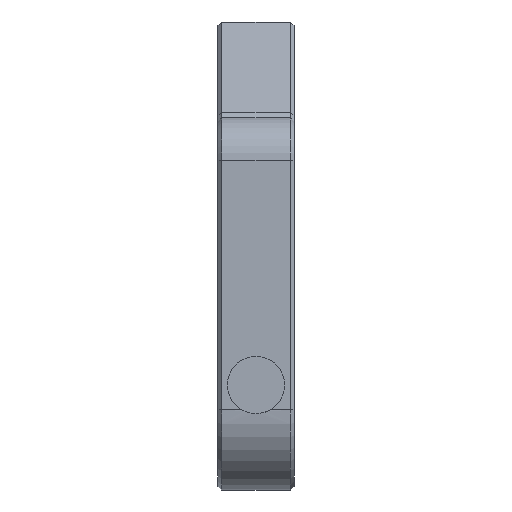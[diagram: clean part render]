
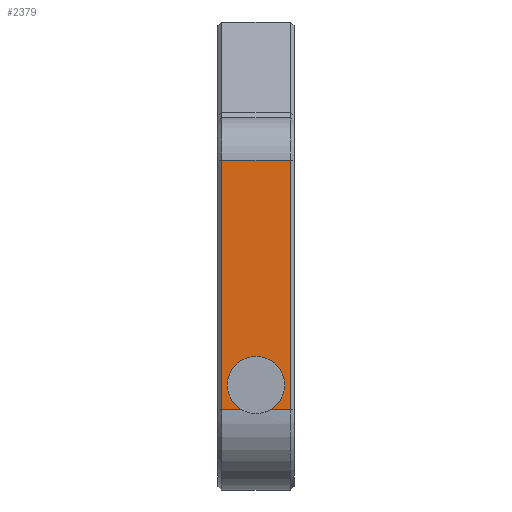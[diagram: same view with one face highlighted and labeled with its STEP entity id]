
A CAD part, left-side view. The second image highlights one B-rep face of the part: STEP entity #2379.
In plain terms, the highlighted planar face has unit normal (-1, 0, 0).
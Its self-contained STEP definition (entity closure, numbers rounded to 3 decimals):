
#224 = PLANE('',#225);
#225 = AXIS2_PLACEMENT_3D('',#226,#227,#228);
#226 = CARTESIAN_POINT('',(11.2,-3.8,-28.5));
#227 = DIRECTION('',(0.707,0.707,0.));
#228 = DIRECTION('',(0.,0.,-1.));
#1197 = VERTEX_POINT('',#1198);
#1198 = CARTESIAN_POINT('',(11.,-3.6,-28.5));
#1232 = CYLINDRICAL_SURFACE('',#1233,4.5);
#1233 = AXIS2_PLACEMENT_3D('',#1234,#1235,#1236);
#1234 = CARTESIAN_POINT('',(15.5,-4.,-28.5));
#1235 = DIRECTION('',(0.,1.,0.));
#1236 = DIRECTION('',(-1.,0.,0.));
#1303 = VERTEX_POINT('',#1304);
#1304 = CARTESIAN_POINT('',(11.,-3.6,-54.6));
#1323 = EDGE_CURVE('',#1197,#1303,#1324,.T.);
#1324 = SURFACE_CURVE('',#1325,(#1329,#1336),.PCURVE_S1.);
#1325 = LINE('',#1326,#1327);
#1326 = CARTESIAN_POINT('',(11.,-3.6,-28.5));
#1327 = VECTOR('',#1328,1.);
#1328 = DIRECTION('',(-0.,-0.,-1.));
#1329 = PCURVE('',#224,#1330);
#1330 = DEFINITIONAL_REPRESENTATION('',(#1331),#1335);
#1331 = LINE('',#1332,#1333);
#1332 = CARTESIAN_POINT('',(0.,0.283));
#1333 = VECTOR('',#1334,1.);
#1334 = DIRECTION('',(1.,0.));
#1335 = ( GEOMETRIC_REPRESENTATION_CONTEXT(2) 
PARAMETRIC_REPRESENTATION_CONTEXT() REPRESENTATION_CONTEXT('2D SPACE',''
  ) );
#1336 = PCURVE('',#1337,#1342);
#1337 = PLANE('',#1338);
#1338 = AXIS2_PLACEMENT_3D('',#1339,#1340,#1341);
#1339 = CARTESIAN_POINT('',(11.,-4.,-63.));
#1340 = DIRECTION('',(1.,0.,0.));
#1341 = DIRECTION('',(0.,0.,1.));
#1342 = DEFINITIONAL_REPRESENTATION('',(#1343),#1347);
#1343 = LINE('',#1344,#1345);
#1344 = CARTESIAN_POINT('',(34.5,-0.4));
#1345 = VECTOR('',#1346,1.);
#1346 = DIRECTION('',(-1.,0.));
#1347 = ( GEOMETRIC_REPRESENTATION_CONTEXT(2) 
PARAMETRIC_REPRESENTATION_CONTEXT() REPRESENTATION_CONTEXT('2D SPACE',''
  ) );
#1443 = CYLINDRICAL_SURFACE('',#1444,8.4);
#1444 = AXIS2_PLACEMENT_3D('',#1445,#1446,#1447);
#1445 = CARTESIAN_POINT('',(19.4,-4.,-54.6));
#1446 = DIRECTION('',(0.,1.,0.));
#1447 = DIRECTION('',(0.,0.,-1.));
#2275 = VERTEX_POINT('',#2276);
#2276 = CARTESIAN_POINT('',(11.,3.6,-28.5));
#2303 = EDGE_CURVE('',#1197,#2275,#2304,.T.);
#2304 = SURFACE_CURVE('',#2305,(#2309,#2316),.PCURVE_S1.);
#2305 = LINE('',#2306,#2307);
#2306 = CARTESIAN_POINT('',(11.,-4.,-28.5));
#2307 = VECTOR('',#2308,1.);
#2308 = DIRECTION('',(0.,1.,0.));
#2309 = PCURVE('',#1232,#2310);
#2310 = DEFINITIONAL_REPRESENTATION('',(#2311),#2315);
#2311 = LINE('',#2312,#2313);
#2312 = CARTESIAN_POINT('',(0.,0.));
#2313 = VECTOR('',#2314,1.);
#2314 = DIRECTION('',(0.,1.));
#2315 = ( GEOMETRIC_REPRESENTATION_CONTEXT(2) 
PARAMETRIC_REPRESENTATION_CONTEXT() REPRESENTATION_CONTEXT('2D SPACE',''
  ) );
#2316 = PCURVE('',#1337,#2317);
#2317 = DEFINITIONAL_REPRESENTATION('',(#2318),#2322);
#2318 = LINE('',#2319,#2320);
#2319 = CARTESIAN_POINT('',(34.5,0.));
#2320 = VECTOR('',#2321,1.);
#2321 = DIRECTION('',(0.,-1.));
#2322 = ( GEOMETRIC_REPRESENTATION_CONTEXT(2) 
PARAMETRIC_REPRESENTATION_CONTEXT() REPRESENTATION_CONTEXT('2D SPACE',''
  ) );
#2379 = ADVANCED_FACE('',(#2380),#1337,.F.);
#2380 = FACE_BOUND('',#2381,.F.);
#2381 = EDGE_LOOP('',(#2382,#2383,#2384,#2407,#2440,#2463));
#2382 = ORIENTED_EDGE('',*,*,#2303,.F.);
#2383 = ORIENTED_EDGE('',*,*,#1323,.T.);
#2384 = ORIENTED_EDGE('',*,*,#2385,.T.);
#2385 = EDGE_CURVE('',#1303,#2386,#2388,.T.);
#2386 = VERTEX_POINT('',#2387);
#2387 = CARTESIAN_POINT('',(11.,-1.497,-54.6));
#2388 = SURFACE_CURVE('',#2389,(#2393,#2400),.PCURVE_S1.);
#2389 = LINE('',#2390,#2391);
#2390 = CARTESIAN_POINT('',(11.,-4.,-54.6));
#2391 = VECTOR('',#2392,1.);
#2392 = DIRECTION('',(0.,1.,0.));
#2393 = PCURVE('',#1337,#2394);
#2394 = DEFINITIONAL_REPRESENTATION('',(#2395),#2399);
#2395 = LINE('',#2396,#2397);
#2396 = CARTESIAN_POINT('',(8.4,0.));
#2397 = VECTOR('',#2398,1.);
#2398 = DIRECTION('',(0.,-1.));
#2399 = ( GEOMETRIC_REPRESENTATION_CONTEXT(2) 
PARAMETRIC_REPRESENTATION_CONTEXT() REPRESENTATION_CONTEXT('2D SPACE',''
  ) );
#2400 = PCURVE('',#1443,#2401);
#2401 = DEFINITIONAL_REPRESENTATION('',(#2402),#2406);
#2402 = LINE('',#2403,#2404);
#2403 = CARTESIAN_POINT('',(1.571,0.));
#2404 = VECTOR('',#2405,1.);
#2405 = DIRECTION('',(0.,1.));
#2406 = ( GEOMETRIC_REPRESENTATION_CONTEXT(2) 
PARAMETRIC_REPRESENTATION_CONTEXT() REPRESENTATION_CONTEXT('2D SPACE',''
  ) );
#2407 = ORIENTED_EDGE('',*,*,#2408,.T.);
#2408 = EDGE_CURVE('',#2386,#2409,#2411,.T.);
#2409 = VERTEX_POINT('',#2410);
#2410 = CARTESIAN_POINT('',(11.,1.497,-54.6));
#2411 = SURFACE_CURVE('',#2412,(#2417,#2428),.PCURVE_S1.);
#2412 = CIRCLE('',#2413,3.);
#2413 = AXIS2_PLACEMENT_3D('',#2414,#2415,#2416);
#2414 = CARTESIAN_POINT('',(11.,0.,-52.));
#2415 = DIRECTION('',(-1.,-0.,0.));
#2416 = DIRECTION('',(0.,0.,-1.));
#2417 = PCURVE('',#1337,#2418);
#2418 = DEFINITIONAL_REPRESENTATION('',(#2419),#2427);
#2419 = ( BOUNDED_CURVE() B_SPLINE_CURVE(2,(#2420,#2421,#2422,#2423,
#2424,#2425,#2426),.UNSPECIFIED.,.T.,.F.) B_SPLINE_CURVE_WITH_KNOTS((1,2
    ,2,2,2,1),(-2.094,0.,2.094,4.189,
6.283,8.378),.UNSPECIFIED.) CURVE() 
GEOMETRIC_REPRESENTATION_ITEM() RATIONAL_B_SPLINE_CURVE((1.,0.5,1.,0.5,
1.,0.5,1.)) REPRESENTATION_ITEM('') );
#2420 = CARTESIAN_POINT('',(8.,-4.));
#2421 = CARTESIAN_POINT('',(8.,1.196));
#2422 = CARTESIAN_POINT('',(12.5,-1.402));
#2423 = CARTESIAN_POINT('',(17.,-4.));
#2424 = CARTESIAN_POINT('',(12.5,-6.598));
#2425 = CARTESIAN_POINT('',(8.,-9.196));
#2426 = CARTESIAN_POINT('',(8.,-4.));
#2427 = ( GEOMETRIC_REPRESENTATION_CONTEXT(2) 
PARAMETRIC_REPRESENTATION_CONTEXT() REPRESENTATION_CONTEXT('2D SPACE',''
  ) );
#2428 = PCURVE('',#2429,#2434);
#2429 = CYLINDRICAL_SURFACE('',#2430,3.);
#2430 = AXIS2_PLACEMENT_3D('',#2431,#2432,#2433);
#2431 = CARTESIAN_POINT('',(3.,0.,-52.));
#2432 = DIRECTION('',(-1.,-0.,0.));
#2433 = DIRECTION('',(0.,0.,-1.));
#2434 = DEFINITIONAL_REPRESENTATION('',(#2435),#2439);
#2435 = LINE('',#2436,#2437);
#2436 = CARTESIAN_POINT('',(-6.283,-8.));
#2437 = VECTOR('',#2438,1.);
#2438 = DIRECTION('',(1.,-0.));
#2439 = ( GEOMETRIC_REPRESENTATION_CONTEXT(2) 
PARAMETRIC_REPRESENTATION_CONTEXT() REPRESENTATION_CONTEXT('2D SPACE',''
  ) );
#2440 = ORIENTED_EDGE('',*,*,#2441,.T.);
#2441 = EDGE_CURVE('',#2409,#2442,#2444,.T.);
#2442 = VERTEX_POINT('',#2443);
#2443 = CARTESIAN_POINT('',(11.,3.6,-54.6));
#2444 = SURFACE_CURVE('',#2445,(#2449,#2456),.PCURVE_S1.);
#2445 = LINE('',#2446,#2447);
#2446 = CARTESIAN_POINT('',(11.,-4.,-54.6));
#2447 = VECTOR('',#2448,1.);
#2448 = DIRECTION('',(0.,1.,0.));
#2449 = PCURVE('',#1337,#2450);
#2450 = DEFINITIONAL_REPRESENTATION('',(#2451),#2455);
#2451 = LINE('',#2452,#2453);
#2452 = CARTESIAN_POINT('',(8.4,0.));
#2453 = VECTOR('',#2454,1.);
#2454 = DIRECTION('',(0.,-1.));
#2455 = ( GEOMETRIC_REPRESENTATION_CONTEXT(2) 
PARAMETRIC_REPRESENTATION_CONTEXT() REPRESENTATION_CONTEXT('2D SPACE',''
  ) );
#2456 = PCURVE('',#1443,#2457);
#2457 = DEFINITIONAL_REPRESENTATION('',(#2458),#2462);
#2458 = LINE('',#2459,#2460);
#2459 = CARTESIAN_POINT('',(1.571,0.));
#2460 = VECTOR('',#2461,1.);
#2461 = DIRECTION('',(0.,1.));
#2462 = ( GEOMETRIC_REPRESENTATION_CONTEXT(2) 
PARAMETRIC_REPRESENTATION_CONTEXT() REPRESENTATION_CONTEXT('2D SPACE',''
  ) );
#2463 = ORIENTED_EDGE('',*,*,#2464,.F.);
#2464 = EDGE_CURVE('',#2275,#2442,#2465,.T.);
#2465 = SURFACE_CURVE('',#2466,(#2470,#2477),.PCURVE_S1.);
#2466 = LINE('',#2467,#2468);
#2467 = CARTESIAN_POINT('',(11.,3.6,-28.5));
#2468 = VECTOR('',#2469,1.);
#2469 = DIRECTION('',(-0.,-0.,-1.));
#2470 = PCURVE('',#1337,#2471);
#2471 = DEFINITIONAL_REPRESENTATION('',(#2472),#2476);
#2472 = LINE('',#2473,#2474);
#2473 = CARTESIAN_POINT('',(34.5,-7.6));
#2474 = VECTOR('',#2475,1.);
#2475 = DIRECTION('',(-1.,0.));
#2476 = ( GEOMETRIC_REPRESENTATION_CONTEXT(2) 
PARAMETRIC_REPRESENTATION_CONTEXT() REPRESENTATION_CONTEXT('2D SPACE',''
  ) );
#2477 = PCURVE('',#2478,#2483);
#2478 = PLANE('',#2479);
#2479 = AXIS2_PLACEMENT_3D('',#2480,#2481,#2482);
#2480 = CARTESIAN_POINT('',(11.2,3.8,-28.5));
#2481 = DIRECTION('',(0.707,-0.707,0.));
#2482 = DIRECTION('',(0.,0.,-1.));
#2483 = DEFINITIONAL_REPRESENTATION('',(#2484),#2488);
#2484 = LINE('',#2485,#2486);
#2485 = CARTESIAN_POINT('',(0.,-0.283));
#2486 = VECTOR('',#2487,1.);
#2487 = DIRECTION('',(1.,0.));
#2488 = ( GEOMETRIC_REPRESENTATION_CONTEXT(2) 
PARAMETRIC_REPRESENTATION_CONTEXT() REPRESENTATION_CONTEXT('2D SPACE',''
  ) );
